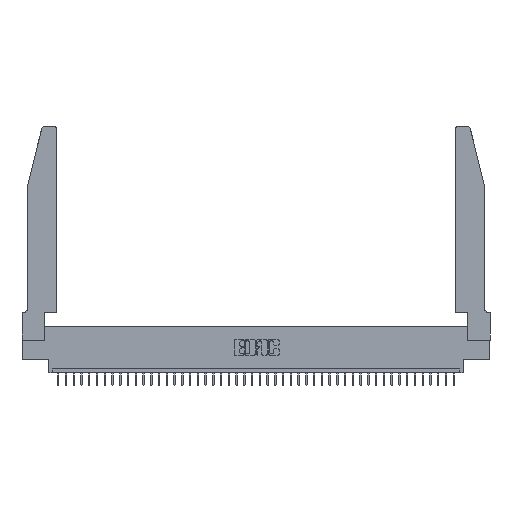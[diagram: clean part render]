
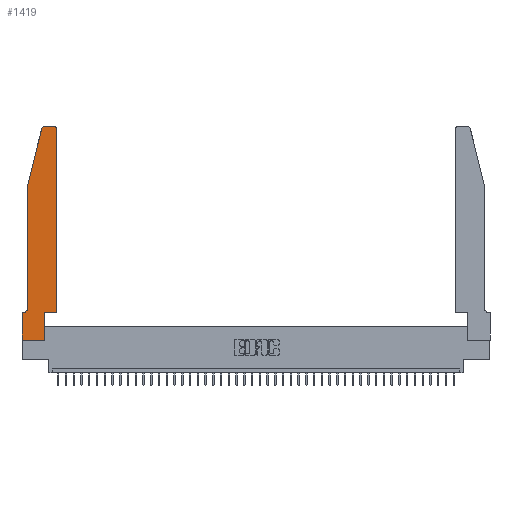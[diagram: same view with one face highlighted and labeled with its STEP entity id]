
A CAD part, top view. The second image highlights one B-rep face of the part: STEP entity #1419.
In plain terms, the highlighted planar face has unit normal (0, 0, 1).
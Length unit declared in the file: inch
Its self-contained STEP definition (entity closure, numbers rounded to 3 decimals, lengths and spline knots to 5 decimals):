
#1360 = EDGE_CURVE ( 'NONE', #37839, #4232, #34172, .T. ) ;
#1400 = CARTESIAN_POINT ( 'NONE',  ( 0.4205, 2.75, 0.37 ) ) ;
#1419 = ADVANCED_FACE ( 'NONE', ( #40895 ), #12737, .T. ) ;
#1795 = VECTOR ( 'NONE', #21346, 39.37008 ) ;
#2287 = LINE ( 'NONE', #40209, #14642 ) ;
#2325 = LINE ( 'NONE', #31090, #1795 ) ;
#2458 = AXIS2_PLACEMENT_3D ( 'NONE', #7023, #30087, #10371 ) ;
#2815 = DIRECTION ( 'NONE',  ( 0., 0., 1. ) ) ;
#2950 = DIRECTION ( 'NONE',  ( 1., 0., 0. ) ) ;
#3373 = VERTEX_POINT ( 'NONE', #23205 ) ;
#4232 = VERTEX_POINT ( 'NONE', #27677 ) ;
#4551 = VECTOR ( 'NONE', #23958, 39.37008 ) ;
#4689 = EDGE_CURVE ( 'NONE', #32533, #5478, #17909, .T. ) ;
#4902 = VECTOR ( 'NONE', #26845, 39.37008 ) ;
#5478 = VERTEX_POINT ( 'NONE', #21157 ) ;
#5903 = EDGE_CURVE ( 'NONE', #5478, #11479, #16723, .T. ) ;
#6071 = EDGE_CURVE ( 'NONE', #33558, #8540, #2325, .T. ) ;
#6440 = ORIENTED_EDGE ( 'NONE', *, *, #11572, .T. ) ;
#6729 = VERTEX_POINT ( 'NONE', #11142 ) ;
#7023 = CARTESIAN_POINT ( 'NONE',  ( 0.284, 2.72, 0.37 ) ) ;
#7242 = CARTESIAN_POINT ( 'NONE',  ( 0.2865, 0., 0.37 ) ) ;
#7273 = DIRECTION ( 'NONE',  ( 0., 0., 1. ) ) ;
#7701 = CARTESIAN_POINT ( 'NONE',  ( 0.0055, 0.35, 0.37 ) ) ;
#7738 = VECTOR ( 'NONE', #40982, 39.37008 ) ;
#8199 = EDGE_CURVE ( 'NONE', #18594, #37839, #41269, .T. ) ;
#8540 = VERTEX_POINT ( 'NONE', #10692 ) ;
#10149 = VECTOR ( 'NONE', #20247, 39.37008 ) ;
#10371 = DIRECTION ( 'NONE',  ( 1., 0., 0. ) ) ;
#10579 = CARTESIAN_POINT ( 'NONE',  ( 0.0755, 0.35, 0.37 ) ) ;
#10692 = CARTESIAN_POINT ( 'NONE',  ( 0.2865, 0.35, 0.37 ) ) ;
#10791 = CARTESIAN_POINT ( 'NONE',  ( 0., 0., 0.37 ) ) ;
#11142 = CARTESIAN_POINT ( 'NONE',  ( 0.4505, 2.72, 0.37 ) ) ;
#11182 = LINE ( 'NONE', #10579, #10149 ) ;
#11479 = VERTEX_POINT ( 'NONE', #7701 ) ;
#11572 = EDGE_CURVE ( 'NONE', #6729, #18594, #14104, .T. ) ;
#12109 = ORIENTED_EDGE ( 'NONE', *, *, #38840, .T. ) ;
#12286 = ORIENTED_EDGE ( 'NONE', *, *, #32452, .T. ) ;
#12305 = EDGE_LOOP ( 'NONE', ( #28800, #39636, #25623, #15738, #16796, #12109, #20420, #21953, #35021, #34173, #12286, #6440 ) ) ;
#12737 = PLANE ( 'NONE',  #42281 ) ;
#14104 = CIRCLE ( 'NONE', #24959, 0.03 ) ;
#14540 = CARTESIAN_POINT ( 'NONE',  ( 0.4505, 0.35, 0.37 ) ) ;
#14642 = VECTOR ( 'NONE', #30064, 39.37008 ) ;
#15718 = VECTOR ( 'NONE', #32914, 39.37008 ) ;
#15738 = ORIENTED_EDGE ( 'NONE', *, *, #4689, .T. ) ;
#16068 = EDGE_CURVE ( 'NONE', #8540, #18935, #28095, .T. ) ;
#16647 = EDGE_CURVE ( 'NONE', #3373, #35289, #2287, .T. ) ;
#16723 = CIRCLE ( 'NONE', #34481, 0.07 ) ;
#16796 = ORIENTED_EDGE ( 'NONE', *, *, #5903, .T. ) ;
#17909 = LINE ( 'NONE', #24704, #38045 ) ;
#18062 = LINE ( 'NONE', #14540, #7738 ) ;
#18344 = DIRECTION ( 'NONE',  ( 0., -1., 0. ) ) ;
#18594 = VERTEX_POINT ( 'NONE', #1400 ) ;
#18935 = VERTEX_POINT ( 'NONE', #29000 ) ;
#20247 = DIRECTION ( 'NONE',  ( -1., 0., 0. ) ) ;
#20420 = ORIENTED_EDGE ( 'NONE', *, *, #16647, .T. ) ;
#21157 = CARTESIAN_POINT ( 'NONE',  ( 0.0755, 0.42, 0.37 ) ) ;
#21346 = DIRECTION ( 'NONE',  ( 0., 1., 0. ) ) ;
#21953 = ORIENTED_EDGE ( 'NONE', *, *, #40238, .T. ) ;
#22130 = LINE ( 'NONE', #24390, #4551 ) ;
#23205 = CARTESIAN_POINT ( 'NONE',  ( 0., 0.35, 0.37 ) ) ;
#23958 = DIRECTION ( 'NONE',  ( 1., 0., 0. ) ) ;
#24079 = CARTESIAN_POINT ( 'NONE',  ( 0.284, 2.75, 0.37 ) ) ;
#24390 = CARTESIAN_POINT ( 'NONE',  ( 0., 0., 0.37 ) ) ;
#24451 = DIRECTION ( 'NONE',  ( 1., 0., 0. ) ) ;
#24704 = CARTESIAN_POINT ( 'NONE',  ( 0.0755, 2., 0.37 ) ) ;
#24959 = AXIS2_PLACEMENT_3D ( 'NONE', #34106, #7273, #24451 ) ;
#25623 = ORIENTED_EDGE ( 'NONE', *, *, #34452, .T. ) ;
#26702 = CARTESIAN_POINT ( 'NONE',  ( 0.4505, 0.35, 0.37 ) ) ;
#26845 = DIRECTION ( 'NONE',  ( 1., 0., 0. ) ) ;
#27677 = CARTESIAN_POINT ( 'NONE',  ( 0.25487, 2.72718, 0.37 ) ) ;
#28095 = LINE ( 'NONE', #26702, #4902 ) ;
#28684 = CARTESIAN_POINT ( 'NONE',  ( 0.2605, 2.75, 0.37 ) ) ;
#28800 = ORIENTED_EDGE ( 'NONE', *, *, #8199, .T. ) ;
#29000 = CARTESIAN_POINT ( 'NONE',  ( 0.4505, 0.35, 0.37 ) ) ;
#29440 = CARTESIAN_POINT ( 'NONE',  ( 0.0755, 2., 0.37 ) ) ;
#30064 = DIRECTION ( 'NONE',  ( 0., -1., 0. ) ) ;
#30087 = DIRECTION ( 'NONE',  ( 0., 0., 1. ) ) ;
#31090 = CARTESIAN_POINT ( 'NONE',  ( 0.2865, 0.35, 0.37 ) ) ;
#31706 = CARTESIAN_POINT ( 'NONE',  ( 0.0755, 2., 0.37 ) ) ;
#32082 = CARTESIAN_POINT ( 'NONE',  ( 0., 0.35, 0.37 ) ) ;
#32156 = DIRECTION ( 'NONE',  ( -1., 0., 0. ) ) ;
#32452 = EDGE_CURVE ( 'NONE', #18935, #6729, #18062, .T. ) ;
#32533 = VERTEX_POINT ( 'NONE', #31706 ) ;
#32914 = DIRECTION ( 'NONE',  ( -0.239, -0.971, 0. ) ) ;
#33558 = VERTEX_POINT ( 'NONE', #7242 ) ;
#34106 = CARTESIAN_POINT ( 'NONE',  ( 0.4205, 2.72, 0.37 ) ) ;
#34172 = CIRCLE ( 'NONE', #2458, 0.03 ) ;
#34173 = ORIENTED_EDGE ( 'NONE', *, *, #16068, .T. ) ;
#34452 = EDGE_CURVE ( 'NONE', #4232, #32533, #36356, .T. ) ;
#34481 = AXIS2_PLACEMENT_3D ( 'NONE', #35691, #36103, #39163 ) ;
#35021 = ORIENTED_EDGE ( 'NONE', *, *, #6071, .T. ) ;
#35289 = VERTEX_POINT ( 'NONE', #10791 ) ;
#35691 = CARTESIAN_POINT ( 'NONE',  ( 0.0055, 0.42, 0.37 ) ) ;
#36103 = DIRECTION ( 'NONE',  ( 0., 0., -1. ) ) ;
#36356 = LINE ( 'NONE', #29440, #15718 ) ;
#37839 = VERTEX_POINT ( 'NONE', #24079 ) ;
#38045 = VECTOR ( 'NONE', #18344, 39.37008 ) ;
#38707 = VECTOR ( 'NONE', #32156, 39.37008 ) ;
#38840 = EDGE_CURVE ( 'NONE', #11479, #3373, #11182, .T. ) ;
#39163 = DIRECTION ( 'NONE',  ( -1., 0., 0. ) ) ;
#39636 = ORIENTED_EDGE ( 'NONE', *, *, #1360, .T. ) ;
#40209 = CARTESIAN_POINT ( 'NONE',  ( 0., 0., 0.37 ) ) ;
#40238 = EDGE_CURVE ( 'NONE', #35289, #33558, #22130, .T. ) ;
#40895 = FACE_OUTER_BOUND ( 'NONE', #12305, .T. ) ;
#40982 = DIRECTION ( 'NONE',  ( 0., 1., 0. ) ) ;
#41269 = LINE ( 'NONE', #28684, #38707 ) ;
#42281 = AXIS2_PLACEMENT_3D ( 'NONE', #32082, #2815, #2950 ) ;
